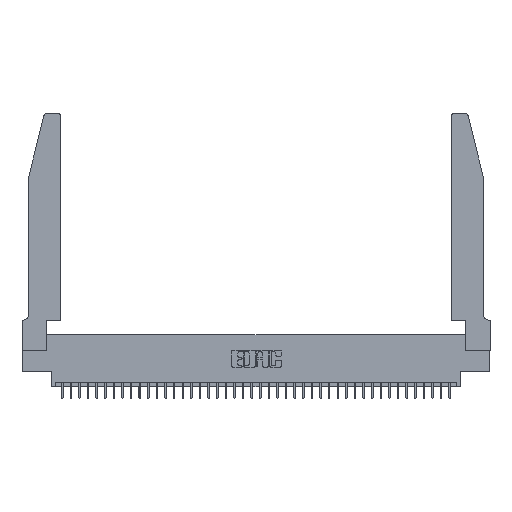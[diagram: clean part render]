
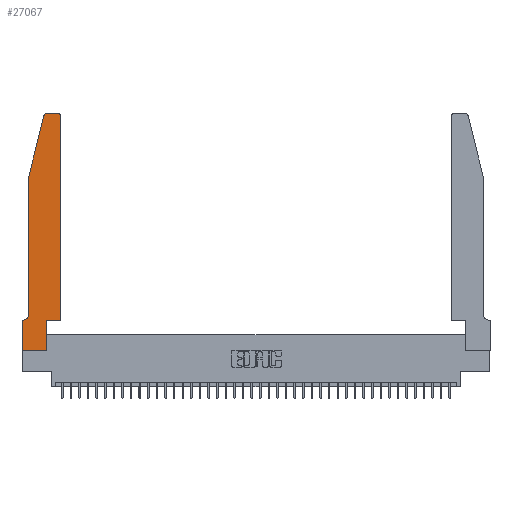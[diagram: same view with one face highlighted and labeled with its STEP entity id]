
A CAD part, top view. The second image highlights one B-rep face of the part: STEP entity #27067.
In plain terms, the highlighted planar face has unit normal (0, 0, 1).
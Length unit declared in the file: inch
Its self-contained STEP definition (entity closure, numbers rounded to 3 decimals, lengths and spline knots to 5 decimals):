
#702 = LINE ( 'NONE', #35188, #26725 ) ;
#712 = CARTESIAN_POINT ( 'NONE',  ( 0.25487, 2.72718, 0.37 ) ) ;
#839 = CARTESIAN_POINT ( 'NONE',  ( 0.0055, 0.42, 0.37 ) ) ;
#1017 = AXIS2_PLACEMENT_3D ( 'NONE', #10380, #32342, #4211 ) ;
#1290 = VECTOR ( 'NONE', #36210, 39.37008 ) ;
#1529 = CARTESIAN_POINT ( 'NONE',  ( 0.4505, 0.35, 0.37 ) ) ;
#1860 = ORIENTED_EDGE ( 'NONE', *, *, #19540, .T. ) ;
#2196 = VERTEX_POINT ( 'NONE', #36261 ) ;
#2652 = EDGE_CURVE ( 'NONE', #30359, #24099, #8103, .T. ) ;
#3117 = VECTOR ( 'NONE', #21190, 39.37008 ) ;
#3212 = ORIENTED_EDGE ( 'NONE', *, *, #33902, .T. ) ;
#3461 = CARTESIAN_POINT ( 'NONE',  ( 0., 0., 0.37 ) ) ;
#3627 = CARTESIAN_POINT ( 'NONE',  ( 0., 0.35, 0.37 ) ) ;
#3735 = VECTOR ( 'NONE', #18131, 39.37008 ) ;
#3807 = ORIENTED_EDGE ( 'NONE', *, *, #17410, .T. ) ;
#4211 = DIRECTION ( 'NONE',  ( 1., 0., 0. ) ) ;
#5103 = CARTESIAN_POINT ( 'NONE',  ( 0.0055, 0.35, 0.37 ) ) ;
#5212 = ORIENTED_EDGE ( 'NONE', *, *, #30344, .T. ) ;
#6669 = ORIENTED_EDGE ( 'NONE', *, *, #15685, .T. ) ;
#6895 = FACE_OUTER_BOUND ( 'NONE', #14548, .T. ) ;
#6960 = VECTOR ( 'NONE', #14191, 39.37008 ) ;
#7061 = DIRECTION ( 'NONE',  ( 0., -1., 0. ) ) ;
#7601 = CARTESIAN_POINT ( 'NONE',  ( 0.2605, 2.75, 0.37 ) ) ;
#7851 = DIRECTION ( 'NONE',  ( 1., 0., 0. ) ) ;
#8103 = LINE ( 'NONE', #1529, #1290 ) ;
#8612 = CARTESIAN_POINT ( 'NONE',  ( 0.2865, 0.35, 0.37 ) ) ;
#9161 = VERTEX_POINT ( 'NONE', #12182 ) ;
#9321 = CARTESIAN_POINT ( 'NONE',  ( 0., 0., 0.37 ) ) ;
#10251 = ORIENTED_EDGE ( 'NONE', *, *, #24881, .T. ) ;
#10269 = DIRECTION ( 'NONE',  ( -1., 0., 0. ) ) ;
#10380 = CARTESIAN_POINT ( 'NONE',  ( 0., 0.35, 0.37 ) ) ;
#10523 = ORIENTED_EDGE ( 'NONE', *, *, #39394, .T. ) ;
#10604 = DIRECTION ( 'NONE',  ( -0.239, -0.971, 0. ) ) ;
#12182 = CARTESIAN_POINT ( 'NONE',  ( 0.4205, 2.75, 0.37 ) ) ;
#13384 = CARTESIAN_POINT ( 'NONE',  ( 0.0755, 0.42, 0.37 ) ) ;
#13593 = CARTESIAN_POINT ( 'NONE',  ( 0., 0., 0.37 ) ) ;
#14109 = DIRECTION ( 'NONE',  ( 1., 0., 0. ) ) ;
#14191 = DIRECTION ( 'NONE',  ( -1., 0., 0. ) ) ;
#14482 = VERTEX_POINT ( 'NONE', #13384 ) ;
#14548 = EDGE_LOOP ( 'NONE', ( #10523, #31857, #5212, #1860, #10251, #6669, #33316, #3212, #38605, #30719, #34205, #3807 ) ) ;
#14790 = CARTESIAN_POINT ( 'NONE',  ( 0.2865, 0., 0.37 ) ) ;
#14805 = LINE ( 'NONE', #31234, #3117 ) ;
#15685 = EDGE_CURVE ( 'NONE', #26163, #17732, #21180, .T. ) ;
#15970 = DIRECTION ( 'NONE',  ( 0., -1., 0. ) ) ;
#16940 = LINE ( 'NONE', #39119, #30495 ) ;
#17410 = EDGE_CURVE ( 'NONE', #2196, #9161, #21383, .T. ) ;
#17732 = VERTEX_POINT ( 'NONE', #3627 ) ;
#18131 = DIRECTION ( 'NONE',  ( 1., 0., 0. ) ) ;
#19540 = EDGE_CURVE ( 'NONE', #29867, #14482, #702, .T. ) ;
#19699 = VECTOR ( 'NONE', #15970, 39.37008 ) ;
#20111 = DIRECTION ( 'NONE',  ( -1., 0., 0. ) ) ;
#20508 = DIRECTION ( 'NONE',  ( 0., 1., 0. ) ) ;
#20972 = VERTEX_POINT ( 'NONE', #13593 ) ;
#20976 = CARTESIAN_POINT ( 'NONE',  ( 0.284, 2.72, 0.37 ) ) ;
#21180 = LINE ( 'NONE', #30604, #6960 ) ;
#21190 = DIRECTION ( 'NONE',  ( 0., 1., 0. ) ) ;
#21255 = EDGE_CURVE ( 'NONE', #17732, #20972, #34670, .T. ) ;
#21383 = CIRCLE ( 'NONE', #29224, 0.03 ) ;
#22366 = EDGE_CURVE ( 'NONE', #36774, #30659, #23058, .T. ) ;
#23058 = CIRCLE ( 'NONE', #40068, 0.03 ) ;
#23408 = LINE ( 'NONE', #7601, #32852 ) ;
#24099 = VERTEX_POINT ( 'NONE', #35935 ) ;
#24271 = DIRECTION ( 'NONE',  ( 0., 0., 1. ) ) ;
#24398 = CARTESIAN_POINT ( 'NONE',  ( 0.0755, 2., 0.37 ) ) ;
#24522 = CIRCLE ( 'NONE', #38250, 0.07 ) ;
#24881 = EDGE_CURVE ( 'NONE', #14482, #26163, #24522, .T. ) ;
#24968 = EDGE_CURVE ( 'NONE', #31251, #30359, #33440, .T. ) ;
#25872 = DIRECTION ( 'NONE',  ( 0., 0., -1. ) ) ;
#26163 = VERTEX_POINT ( 'NONE', #5103 ) ;
#26725 = VECTOR ( 'NONE', #7061, 39.37008 ) ;
#27067 = ADVANCED_FACE ( 'NONE', ( #6895 ), #38892, .T. ) ;
#27546 = CARTESIAN_POINT ( 'NONE',  ( 0.284, 2.75, 0.37 ) ) ;
#29224 = AXIS2_PLACEMENT_3D ( 'NONE', #35878, #39347, #14109 ) ;
#29867 = VERTEX_POINT ( 'NONE', #24398 ) ;
#29875 = CARTESIAN_POINT ( 'NONE',  ( 0.2865, 0.35, 0.37 ) ) ;
#30344 = EDGE_CURVE ( 'NONE', #30659, #29867, #16940, .T. ) ;
#30359 = VERTEX_POINT ( 'NONE', #29875 ) ;
#30495 = VECTOR ( 'NONE', #10604, 39.37008 ) ;
#30604 = CARTESIAN_POINT ( 'NONE',  ( 0.0755, 0.35, 0.37 ) ) ;
#30659 = VERTEX_POINT ( 'NONE', #712 ) ;
#30719 = ORIENTED_EDGE ( 'NONE', *, *, #2652, .T. ) ;
#31039 = VECTOR ( 'NONE', #20508, 39.37008 ) ;
#31234 = CARTESIAN_POINT ( 'NONE',  ( 0.4505, 0.35, 0.37 ) ) ;
#31251 = VERTEX_POINT ( 'NONE', #14790 ) ;
#31857 = ORIENTED_EDGE ( 'NONE', *, *, #22366, .T. ) ;
#32342 = DIRECTION ( 'NONE',  ( 0., 0., 1. ) ) ;
#32852 = VECTOR ( 'NONE', #20111, 39.37008 ) ;
#33316 = ORIENTED_EDGE ( 'NONE', *, *, #21255, .T. ) ;
#33440 = LINE ( 'NONE', #8612, #31039 ) ;
#33902 = EDGE_CURVE ( 'NONE', #20972, #31251, #37423, .T. ) ;
#34205 = ORIENTED_EDGE ( 'NONE', *, *, #35428, .T. ) ;
#34670 = LINE ( 'NONE', #3461, #19699 ) ;
#35188 = CARTESIAN_POINT ( 'NONE',  ( 0.0755, 2., 0.37 ) ) ;
#35428 = EDGE_CURVE ( 'NONE', #24099, #2196, #14805, .T. ) ;
#35878 = CARTESIAN_POINT ( 'NONE',  ( 0.4205, 2.72, 0.37 ) ) ;
#35935 = CARTESIAN_POINT ( 'NONE',  ( 0.4505, 0.35, 0.37 ) ) ;
#36210 = DIRECTION ( 'NONE',  ( 1., 0., 0. ) ) ;
#36261 = CARTESIAN_POINT ( 'NONE',  ( 0.4505, 2.72, 0.37 ) ) ;
#36774 = VERTEX_POINT ( 'NONE', #27546 ) ;
#37423 = LINE ( 'NONE', #9321, #3735 ) ;
#38250 = AXIS2_PLACEMENT_3D ( 'NONE', #839, #25872, #10269 ) ;
#38605 = ORIENTED_EDGE ( 'NONE', *, *, #24968, .T. ) ;
#38892 = PLANE ( 'NONE',  #1017 ) ;
#39119 = CARTESIAN_POINT ( 'NONE',  ( 0.0755, 2., 0.37 ) ) ;
#39347 = DIRECTION ( 'NONE',  ( 0., 0., 1. ) ) ;
#39394 = EDGE_CURVE ( 'NONE', #9161, #36774, #23408, .T. ) ;
#40068 = AXIS2_PLACEMENT_3D ( 'NONE', #20976, #24271, #7851 ) ;
